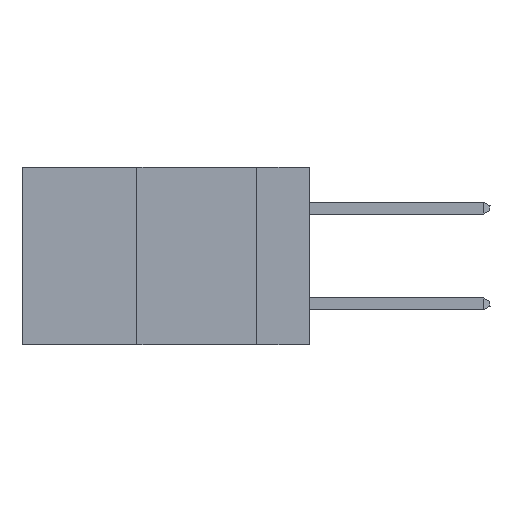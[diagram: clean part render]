
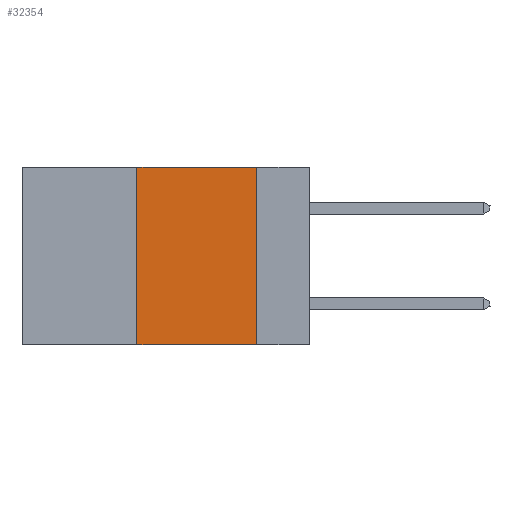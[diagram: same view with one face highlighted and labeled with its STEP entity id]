
A CAD part, left-side view. The second image highlights one B-rep face of the part: STEP entity #32354.
In plain terms, the highlighted planar face has unit normal (-1, 0, 0).
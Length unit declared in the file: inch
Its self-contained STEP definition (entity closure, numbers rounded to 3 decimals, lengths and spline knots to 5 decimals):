
#95 = LINE ( 'NONE', #42691, #34786 ) ;
#689 = CARTESIAN_POINT ( 'NONE',  ( 0., 0.11, 0. ) ) ;
#1454 = VECTOR ( 'NONE', #34753, 39.37008 ) ;
#1551 = VERTEX_POINT ( 'NONE', #9404 ) ;
#5060 = EDGE_CURVE ( 'NONE', #15586, #32500, #95, .T. ) ;
#5656 = LINE ( 'NONE', #689, #1454 ) ;
#6489 = CARTESIAN_POINT ( 'NONE',  ( 0., 0.6, -0.37 ) ) ;
#9404 = CARTESIAN_POINT ( 'NONE',  ( 0., 0.11, -0.37 ) ) ;
#11916 = AXIS2_PLACEMENT_3D ( 'NONE', #33560, #23722, #20469 ) ;
#14033 = VERTEX_POINT ( 'NONE', #39006 ) ;
#14174 = CARTESIAN_POINT ( 'NONE',  ( 0., 0.36, -0.37 ) ) ;
#14256 = LINE ( 'NONE', #6489, #16405 ) ;
#14542 = DIRECTION ( 'NONE',  ( 0., -1., 0. ) ) ;
#15586 = VERTEX_POINT ( 'NONE', #14174 ) ;
#16399 = EDGE_CURVE ( 'NONE', #15586, #1551, #14256, .T. ) ;
#16405 = VECTOR ( 'NONE', #40282, 39.37008 ) ;
#16626 = ORIENTED_EDGE ( 'NONE', *, *, #39657, .F. ) ;
#17852 = ORIENTED_EDGE ( 'NONE', *, *, #5060, .F. ) ;
#17986 = ORIENTED_EDGE ( 'NONE', *, *, #35618, .F. ) ;
#18607 = EDGE_LOOP ( 'NONE', ( #17986, #16626, #17852, #36545 ) ) ;
#20469 = DIRECTION ( 'NONE',  ( 0., 0., -1. ) ) ;
#22676 = LINE ( 'NONE', #31286, #39500 ) ;
#23722 = DIRECTION ( 'NONE',  ( 1., 0., 0. ) ) ;
#29445 = DIRECTION ( 'NONE',  ( 0., 0., 1. ) ) ;
#29978 = FACE_OUTER_BOUND ( 'NONE', #18607, .T. ) ;
#31286 = CARTESIAN_POINT ( 'NONE',  ( 0., 0.6, 0. ) ) ;
#32354 = ADVANCED_FACE ( 'NONE', ( #29978 ), #33851, .F. ) ;
#32500 = VERTEX_POINT ( 'NONE', #41574 ) ;
#33560 = CARTESIAN_POINT ( 'NONE',  ( 0., 0.6, 0. ) ) ;
#33851 = PLANE ( 'NONE',  #11916 ) ;
#34753 = DIRECTION ( 'NONE',  ( 0., 0., -1. ) ) ;
#34786 = VECTOR ( 'NONE', #29445, 39.37008 ) ;
#35618 = EDGE_CURVE ( 'NONE', #14033, #1551, #5656, .T. ) ;
#36545 = ORIENTED_EDGE ( 'NONE', *, *, #16399, .T. ) ;
#39006 = CARTESIAN_POINT ( 'NONE',  ( 0., 0.11, 0. ) ) ;
#39500 = VECTOR ( 'NONE', #14542, 39.37008 ) ;
#39657 = EDGE_CURVE ( 'NONE', #32500, #14033, #22676, .T. ) ;
#40282 = DIRECTION ( 'NONE',  ( 0., -1., 0. ) ) ;
#41574 = CARTESIAN_POINT ( 'NONE',  ( 0., 0.36, 0. ) ) ;
#42691 = CARTESIAN_POINT ( 'NONE',  ( 0., 0.36, 0. ) ) ;
